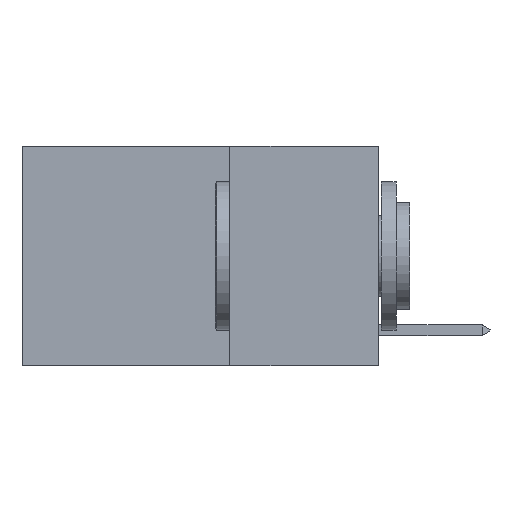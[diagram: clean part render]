
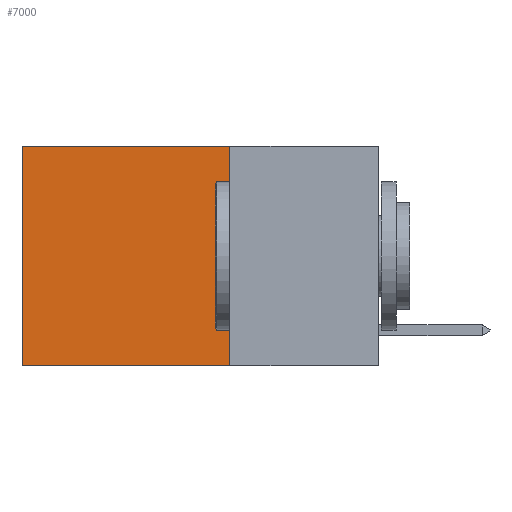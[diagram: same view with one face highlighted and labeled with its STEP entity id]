
A CAD part, left-side view. The second image highlights one B-rep face of the part: STEP entity #7000.
In plain terms, the highlighted planar face has unit normal (-1, 0, 0).
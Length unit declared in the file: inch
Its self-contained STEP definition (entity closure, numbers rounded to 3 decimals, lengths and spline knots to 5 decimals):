
#1199 = CARTESIAN_POINT ( 'NONE',  ( 0.2625, 0.25, 0. ) ) ;
#1608 = DIRECTION ( 'NONE',  ( 1., 0., 0. ) ) ;
#1780 = ORIENTED_EDGE ( 'NONE', *, *, #15241, .F. ) ;
#2278 = VECTOR ( 'NONE', #26193, 39.37008 ) ;
#2338 = DIRECTION ( 'NONE',  ( 0., 0., -1. ) ) ;
#2462 = EDGE_CURVE ( 'NONE', #16577, #2624, #3445, .T. ) ;
#2624 = VERTEX_POINT ( 'NONE', #4116 ) ;
#3445 = LINE ( 'NONE', #25927, #17017 ) ;
#4116 = CARTESIAN_POINT ( 'NONE',  ( 0.2625, 0.6, 0. ) ) ;
#4611 = CARTESIAN_POINT ( 'NONE',  ( 0.2625, 0.25, -0.37 ) ) ;
#4915 = CARTESIAN_POINT ( 'NONE',  ( 0.2625, 0.25, -0.37 ) ) ;
#7000 = ADVANCED_FACE ( 'NONE', ( #11512 ), #19774, .F. ) ;
#7175 = VECTOR ( 'NONE', #2338, 39.37008 ) ;
#8403 = LINE ( 'NONE', #4611, #8640 ) ;
#8640 = VECTOR ( 'NONE', #22776, 39.37008 ) ;
#9300 = DIRECTION ( 'NONE',  ( 0., 1., 0. ) ) ;
#10342 = LINE ( 'NONE', #18603, #7175 ) ;
#11273 = EDGE_CURVE ( 'NONE', #24999, #13352, #8403, .T. ) ;
#11512 = FACE_OUTER_BOUND ( 'NONE', #23530, .T. ) ;
#13352 = VERTEX_POINT ( 'NONE', #24195 ) ;
#13825 = ORIENTED_EDGE ( 'NONE', *, *, #2462, .T. ) ;
#15241 = EDGE_CURVE ( 'NONE', #16577, #24999, #10342, .T. ) ;
#15506 = AXIS2_PLACEMENT_3D ( 'NONE', #1199, #1608, #16636 ) ;
#16066 = ORIENTED_EDGE ( 'NONE', *, *, #11273, .F. ) ;
#16577 = VERTEX_POINT ( 'NONE', #23012 ) ;
#16636 = DIRECTION ( 'NONE',  ( 0., 0., -1. ) ) ;
#17017 = VECTOR ( 'NONE', #9300, 39.37008 ) ;
#17948 = CARTESIAN_POINT ( 'NONE',  ( 0.2625, 0.6, 0. ) ) ;
#18603 = CARTESIAN_POINT ( 'NONE',  ( 0.2625, 0.25, 0. ) ) ;
#18730 = EDGE_CURVE ( 'NONE', #2624, #13352, #19981, .T. ) ;
#19774 = PLANE ( 'NONE',  #15506 ) ;
#19981 = LINE ( 'NONE', #17948, #2278 ) ;
#20630 = ORIENTED_EDGE ( 'NONE', *, *, #18730, .T. ) ;
#22776 = DIRECTION ( 'NONE',  ( 0., 1., 0. ) ) ;
#23012 = CARTESIAN_POINT ( 'NONE',  ( 0.2625, 0.25, 0. ) ) ;
#23530 = EDGE_LOOP ( 'NONE', ( #20630, #16066, #1780, #13825 ) ) ;
#24195 = CARTESIAN_POINT ( 'NONE',  ( 0.2625, 0.6, -0.37 ) ) ;
#24999 = VERTEX_POINT ( 'NONE', #4915 ) ;
#25927 = CARTESIAN_POINT ( 'NONE',  ( 0.2625, 0.25, 0. ) ) ;
#26193 = DIRECTION ( 'NONE',  ( 0., 0., -1. ) ) ;
